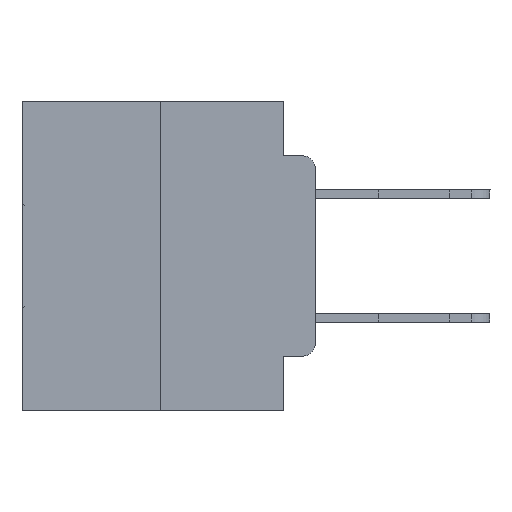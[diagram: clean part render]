
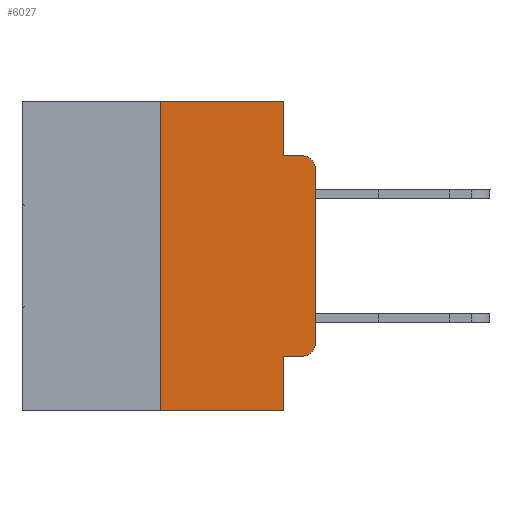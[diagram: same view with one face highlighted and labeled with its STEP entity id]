
A CAD part, left-side view. The second image highlights one B-rep face of the part: STEP entity #6027.
In plain terms, the highlighted planar face has unit normal (-1, 0, 0).
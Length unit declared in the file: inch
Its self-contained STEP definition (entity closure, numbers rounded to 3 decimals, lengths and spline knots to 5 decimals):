
#852 = EDGE_CURVE ( 'NONE', #13304, #5409, #9121, .T. ) ;
#1267 = EDGE_CURVE ( 'NONE', #6862, #11497, #21118, .T. ) ;
#1306 = CARTESIAN_POINT ( 'NONE',  ( 0., 0.25, -0.5 ) ) ;
#1610 = CARTESIAN_POINT ( 'NONE',  ( 0., 0.051, -0.5 ) ) ;
#1656 = CARTESIAN_POINT ( 'NONE',  ( 0., 0.051, -0.4115 ) ) ;
#1806 = AXIS2_PLACEMENT_3D ( 'NONE', #2293, #27523, #6958 ) ;
#2161 = CARTESIAN_POINT ( 'NONE',  ( 0., 0., -0.1085 ) ) ;
#2293 = CARTESIAN_POINT ( 'NONE',  ( 0., 0.02, -0.3915 ) ) ;
#2361 = EDGE_CURVE ( 'NONE', #10649, #16370, #19192, .T. ) ;
#2534 = DIRECTION ( 'NONE',  ( 0., 0., 1. ) ) ;
#2667 = VECTOR ( 'NONE', #25204, 39.37008 ) ;
#2891 = ORIENTED_EDGE ( 'NONE', *, *, #4806, .T. ) ;
#3694 = ORIENTED_EDGE ( 'NONE', *, *, #4984, .T. ) ;
#4398 = ORIENTED_EDGE ( 'NONE', *, *, #15986, .T. ) ;
#4806 = EDGE_CURVE ( 'NONE', #13115, #29239, #6016, .T. ) ;
#4984 = EDGE_CURVE ( 'NONE', #11497, #16370, #19946, .T. ) ;
#5409 = VERTEX_POINT ( 'NONE', #14056 ) ;
#5423 = DIRECTION ( 'NONE',  ( 1., 0., 0. ) ) ;
#5493 = EDGE_CURVE ( 'NONE', #10918, #21936, #15078, .T. ) ;
#5870 = CARTESIAN_POINT ( 'NONE',  ( 0., 0.473, 0. ) ) ;
#6016 = LINE ( 'NONE', #1656, #27994 ) ;
#6027 = ADVANCED_FACE ( 'NONE', ( #26010 ), #8106, .F. ) ;
#6034 = ORIENTED_EDGE ( 'NONE', *, *, #26480, .F. ) ;
#6604 = ORIENTED_EDGE ( 'NONE', *, *, #5493, .T. ) ;
#6862 = VERTEX_POINT ( 'NONE', #21441 ) ;
#6878 = CARTESIAN_POINT ( 'NONE',  ( 0., 0.473, 0. ) ) ;
#6902 = DIRECTION ( 'NONE',  ( -1., 0., 0. ) ) ;
#6958 = DIRECTION ( 'NONE',  ( 0., 0., -1. ) ) ;
#7040 = VECTOR ( 'NONE', #18412, 39.37008 ) ;
#7639 = VECTOR ( 'NONE', #23799, 39.37008 ) ;
#7749 = CARTESIAN_POINT ( 'NONE',  ( 0., 0.02, -0.4115 ) ) ;
#8106 = PLANE ( 'NONE',  #11364 ) ;
#9121 = LINE ( 'NONE', #6878, #2667 ) ;
#9147 = CARTESIAN_POINT ( 'NONE',  ( 0., 0.02, -0.1085 ) ) ;
#9698 = CARTESIAN_POINT ( 'NONE',  ( 0., 0.051, -0.4115 ) ) ;
#9999 = DIRECTION ( 'NONE',  ( 0., 0., -1. ) ) ;
#10620 = EDGE_CURVE ( 'NONE', #10918, #13304, #22825, .T. ) ;
#10649 = VERTEX_POINT ( 'NONE', #20868 ) ;
#10918 = VERTEX_POINT ( 'NONE', #1306 ) ;
#10955 = DIRECTION ( 'NONE',  ( 0., -1., 0. ) ) ;
#11364 = AXIS2_PLACEMENT_3D ( 'NONE', #5870, #5423, #17287 ) ;
#11497 = VERTEX_POINT ( 'NONE', #2161 ) ;
#11563 = DIRECTION ( 'NONE',  ( 0., 0., -1. ) ) ;
#12709 = LINE ( 'NONE', #21737, #27226 ) ;
#12818 = CARTESIAN_POINT ( 'NONE',  ( 0., 0.473, -0.5 ) ) ;
#13115 = VERTEX_POINT ( 'NONE', #9698 ) ;
#13304 = VERTEX_POINT ( 'NONE', #22756 ) ;
#14056 = CARTESIAN_POINT ( 'NONE',  ( 0., 0.051, 0. ) ) ;
#14138 = VECTOR ( 'NONE', #2534, 39.37008 ) ;
#14447 = LINE ( 'NONE', #20909, #23144 ) ;
#14702 = CARTESIAN_POINT ( 'NONE',  ( 0., 0.051, -0.0885 ) ) ;
#15078 = LINE ( 'NONE', #12818, #7639 ) ;
#15260 = CIRCLE ( 'NONE', #1806, 0.02 ) ;
#15347 = CARTESIAN_POINT ( 'NONE',  ( 0., 0.02, -0.0885 ) ) ;
#15548 = VECTOR ( 'NONE', #19484, 39.37008 ) ;
#15665 = EDGE_CURVE ( 'NONE', #5409, #10649, #12709, .T. ) ;
#15986 = EDGE_CURVE ( 'NONE', #29239, #6862, #15260, .T. ) ;
#16370 = VERTEX_POINT ( 'NONE', #15347 ) ;
#17287 = DIRECTION ( 'NONE',  ( 0., 0., -1. ) ) ;
#17740 = ORIENTED_EDGE ( 'NONE', *, *, #852, .F. ) ;
#18412 = DIRECTION ( 'NONE',  ( 0., 0., 1. ) ) ;
#19192 = LINE ( 'NONE', #14702, #15548 ) ;
#19484 = DIRECTION ( 'NONE',  ( 0., -1., 0. ) ) ;
#19658 = ORIENTED_EDGE ( 'NONE', *, *, #10620, .F. ) ;
#19946 = CIRCLE ( 'NONE', #27615, 0.02 ) ;
#20868 = CARTESIAN_POINT ( 'NONE',  ( 0., 0.051, -0.0885 ) ) ;
#20909 = CARTESIAN_POINT ( 'NONE',  ( 0., 0.051, 0. ) ) ;
#21058 = DIRECTION ( 'NONE',  ( 0., 0., -1. ) ) ;
#21118 = LINE ( 'NONE', #22933, #7040 ) ;
#21441 = CARTESIAN_POINT ( 'NONE',  ( 0., 0., -0.3915 ) ) ;
#21682 = EDGE_LOOP ( 'NONE', ( #23430, #3694, #27144, #28266, #17740, #19658, #6604, #6034, #2891, #4398 ) ) ;
#21737 = CARTESIAN_POINT ( 'NONE',  ( 0., 0.051, 0. ) ) ;
#21936 = VERTEX_POINT ( 'NONE', #1610 ) ;
#22756 = CARTESIAN_POINT ( 'NONE',  ( 0., 0.25, 0. ) ) ;
#22825 = LINE ( 'NONE', #25517, #14138 ) ;
#22933 = CARTESIAN_POINT ( 'NONE',  ( 0., 0., 0. ) ) ;
#23144 = VECTOR ( 'NONE', #21058, 39.37008 ) ;
#23430 = ORIENTED_EDGE ( 'NONE', *, *, #1267, .T. ) ;
#23799 = DIRECTION ( 'NONE',  ( 0., -1., 0. ) ) ;
#25204 = DIRECTION ( 'NONE',  ( 0., -1., 0. ) ) ;
#25517 = CARTESIAN_POINT ( 'NONE',  ( 0., 0.25, 0. ) ) ;
#26010 = FACE_OUTER_BOUND ( 'NONE', #21682, .T. ) ;
#26480 = EDGE_CURVE ( 'NONE', #13115, #21936, #14447, .T. ) ;
#27144 = ORIENTED_EDGE ( 'NONE', *, *, #2361, .F. ) ;
#27226 = VECTOR ( 'NONE', #9999, 39.37008 ) ;
#27523 = DIRECTION ( 'NONE',  ( -1., 0., 0. ) ) ;
#27615 = AXIS2_PLACEMENT_3D ( 'NONE', #9147, #6902, #11563 ) ;
#27994 = VECTOR ( 'NONE', #10955, 39.37008 ) ;
#28266 = ORIENTED_EDGE ( 'NONE', *, *, #15665, .F. ) ;
#29239 = VERTEX_POINT ( 'NONE', #7749 ) ;
